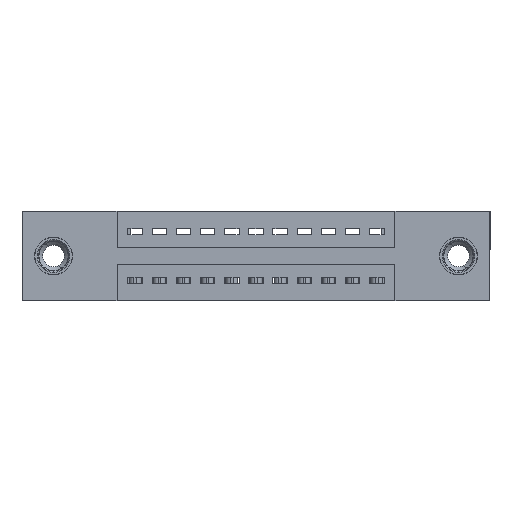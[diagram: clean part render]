
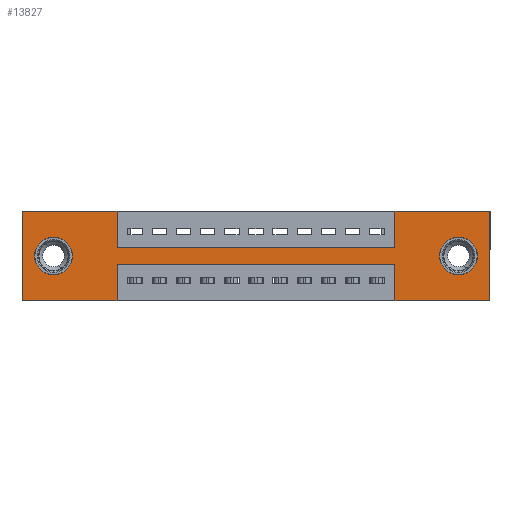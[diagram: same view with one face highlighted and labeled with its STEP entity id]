
A CAD part, front view. The second image highlights one B-rep face of the part: STEP entity #13827.
In plain terms, the highlighted planar face has unit normal (0, -1, 0).
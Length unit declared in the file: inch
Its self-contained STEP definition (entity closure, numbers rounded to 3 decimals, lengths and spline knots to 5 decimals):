
#145 = CARTESIAN_POINT ( 'NONE',  ( 0., 0., -0.37 ) ) ;
#347 = ORIENTED_EDGE ( 'NONE', *, *, #14612, .T. ) ;
#535 = CARTESIAN_POINT ( 'NONE',  ( 1.805, 0., -0.185 ) ) ;
#588 = LINE ( 'NONE', #3285, #9502 ) ;
#739 = ORIENTED_EDGE ( 'NONE', *, *, #3452, .F. ) ;
#837 = EDGE_CURVE ( 'NONE', #3271, #6116, #16174, .T. ) ;
#851 = FACE_BOUND ( 'NONE', #16151, .T. ) ;
#891 = VERTEX_POINT ( 'NONE', #9040 ) ;
#988 = AXIS2_PLACEMENT_3D ( 'NONE', #5003, #3527, #16851 ) ;
#1136 = EDGE_CURVE ( 'NONE', #15679, #12880, #14702, .T. ) ;
#1168 = ORIENTED_EDGE ( 'NONE', *, *, #8587, .F. ) ;
#1301 = ORIENTED_EDGE ( 'NONE', *, *, #837, .F. ) ;
#1637 = CIRCLE ( 'NONE', #9508, 0.078 ) ;
#1881 = DIRECTION ( 'NONE',  ( 0., 1., 0. ) ) ;
#2131 = LINE ( 'NONE', #10244, #5858 ) ;
#2221 = DIRECTION ( 'NONE',  ( 0., 0., 1. ) ) ;
#2283 = VERTEX_POINT ( 'NONE', #6442 ) ;
#2339 = DIRECTION ( 'NONE',  ( 1., 0., 0. ) ) ;
#2840 = CARTESIAN_POINT ( 'NONE',  ( 0.3925, 0., -0.22 ) ) ;
#2903 = VERTEX_POINT ( 'NONE', #14888 ) ;
#2966 = CIRCLE ( 'NONE', #988, 0.078 ) ;
#3119 = CARTESIAN_POINT ( 'NONE',  ( 1.5425, 0., 0. ) ) ;
#3271 = VERTEX_POINT ( 'NONE', #4551 ) ;
#3276 = VERTEX_POINT ( 'NONE', #3298 ) ;
#3285 = CARTESIAN_POINT ( 'NONE',  ( 0.3925, 0., -0.15 ) ) ;
#3298 = CARTESIAN_POINT ( 'NONE',  ( 1.935, 0., -0.37 ) ) ;
#3301 = VERTEX_POINT ( 'NONE', #7769 ) ;
#3452 = EDGE_CURVE ( 'NONE', #891, #11376, #14467, .T. ) ;
#3463 = VECTOR ( 'NONE', #6060, 39.37008 ) ;
#3464 = LINE ( 'NONE', #3119, #4306 ) ;
#3527 = DIRECTION ( 'NONE',  ( 0., 1., 0. ) ) ;
#3656 = CARTESIAN_POINT ( 'NONE',  ( 0., 0., 0. ) ) ;
#3719 = ORIENTED_EDGE ( 'NONE', *, *, #5097, .F. ) ;
#3980 = EDGE_CURVE ( 'NONE', #2903, #5369, #588, .T. ) ;
#4088 = AXIS2_PLACEMENT_3D ( 'NONE', #11231, #12557, #16885 ) ;
#4231 = VECTOR ( 'NONE', #11569, 39.37008 ) ;
#4254 = DIRECTION ( 'NONE',  ( 0., 0., 1. ) ) ;
#4306 = VECTOR ( 'NONE', #4254, 39.37008 ) ;
#4396 = CARTESIAN_POINT ( 'NONE',  ( 0.3925, 0., -0.22 ) ) ;
#4400 = ORIENTED_EDGE ( 'NONE', *, *, #10268, .F. ) ;
#4551 = CARTESIAN_POINT ( 'NONE',  ( 0., 0., 0. ) ) ;
#4624 = VECTOR ( 'NONE', #12164, 39.37008 ) ;
#4629 = ORIENTED_EDGE ( 'NONE', *, *, #10892, .F. ) ;
#4872 = PLANE ( 'NONE',  #4088 ) ;
#5003 = CARTESIAN_POINT ( 'NONE',  ( 0.13, 0., -0.185 ) ) ;
#5087 = VECTOR ( 'NONE', #11631, 39.37008 ) ;
#5097 = EDGE_CURVE ( 'NONE', #11376, #3301, #11520, .T. ) ;
#5207 = CARTESIAN_POINT ( 'NONE',  ( 0.13, 0., -0.107 ) ) ;
#5263 = EDGE_CURVE ( 'NONE', #5369, #9831, #3464, .T. ) ;
#5315 = ORIENTED_EDGE ( 'NONE', *, *, #3980, .F. ) ;
#5369 = VERTEX_POINT ( 'NONE', #14026 ) ;
#5533 = VERTEX_POINT ( 'NONE', #7698 ) ;
#5627 = DIRECTION ( 'NONE',  ( -1., 0., 0. ) ) ;
#5721 = CARTESIAN_POINT ( 'NONE',  ( 1.805, 0., -0.185 ) ) ;
#5858 = VECTOR ( 'NONE', #11624, 39.37008 ) ;
#5893 = ORIENTED_EDGE ( 'NONE', *, *, #1136, .T. ) ;
#5897 = CARTESIAN_POINT ( 'NONE',  ( 1.5425, 0., 0. ) ) ;
#5966 = DIRECTION ( 'NONE',  ( 0., 0., -1. ) ) ;
#6060 = DIRECTION ( 'NONE',  ( 0., 0., -1. ) ) ;
#6116 = VERTEX_POINT ( 'NONE', #10850 ) ;
#6301 = VERTEX_POINT ( 'NONE', #16018 ) ;
#6442 = CARTESIAN_POINT ( 'NONE',  ( 0., 0., -0.37 ) ) ;
#6686 = DIRECTION ( 'NONE',  ( 0., 0., -1. ) ) ;
#7029 = EDGE_CURVE ( 'NONE', #16158, #5533, #15606, .T. ) ;
#7040 = CARTESIAN_POINT ( 'NONE',  ( 1.935, 0., 0. ) ) ;
#7057 = CARTESIAN_POINT ( 'NONE',  ( 1.5425, 0., -0.37 ) ) ;
#7170 = VECTOR ( 'NONE', #2221, 39.37008 ) ;
#7318 = FACE_BOUND ( 'NONE', #10980, .T. ) ;
#7380 = CARTESIAN_POINT ( 'NONE',  ( 0., 0., 0. ) ) ;
#7698 = CARTESIAN_POINT ( 'NONE',  ( 1.805, 0., -0.263 ) ) ;
#7764 = EDGE_CURVE ( 'NONE', #6301, #891, #8377, .T. ) ;
#7769 = CARTESIAN_POINT ( 'NONE',  ( 0.3925, 0., -0.37 ) ) ;
#8266 = CARTESIAN_POINT ( 'NONE',  ( 0.13, 0., -0.185 ) ) ;
#8377 = LINE ( 'NONE', #7057, #13283 ) ;
#8478 = CARTESIAN_POINT ( 'NONE',  ( 0., 0., 0. ) ) ;
#8587 = EDGE_CURVE ( 'NONE', #3301, #2283, #17018, .T. ) ;
#8606 = LINE ( 'NONE', #7380, #7170 ) ;
#8655 = VECTOR ( 'NONE', #6686, 39.37008 ) ;
#9040 = CARTESIAN_POINT ( 'NONE',  ( 1.5425, 0., -0.22 ) ) ;
#9500 = CARTESIAN_POINT ( 'NONE',  ( 0.13, 0., -0.263 ) ) ;
#9502 = VECTOR ( 'NONE', #11256, 39.37008 ) ;
#9508 = AXIS2_PLACEMENT_3D ( 'NONE', #535, #1881, #5966 ) ;
#9686 = DIRECTION ( 'NONE',  ( 0., 0., 1. ) ) ;
#9746 = DIRECTION ( 'NONE',  ( 0., 0., -1. ) ) ;
#9831 = VERTEX_POINT ( 'NONE', #5897 ) ;
#10244 = CARTESIAN_POINT ( 'NONE',  ( 1.935, 0., 0. ) ) ;
#10268 = EDGE_CURVE ( 'NONE', #6116, #2903, #10880, .T. ) ;
#10292 = ORIENTED_EDGE ( 'NONE', *, *, #16569, .T. ) ;
#10850 = CARTESIAN_POINT ( 'NONE',  ( 0.3925, 0., 0. ) ) ;
#10880 = LINE ( 'NONE', #13743, #3463 ) ;
#10892 = EDGE_CURVE ( 'NONE', #2283, #3271, #8606, .T. ) ;
#10980 = EDGE_LOOP ( 'NONE', ( #5893, #10292 ) ) ;
#11017 = DIRECTION ( 'NONE',  ( 0., 0., 1. ) ) ;
#11073 = DIRECTION ( 'NONE',  ( 0., 1., 0. ) ) ;
#11231 = CARTESIAN_POINT ( 'NONE',  ( 0., 0., -0.37 ) ) ;
#11256 = DIRECTION ( 'NONE',  ( 1., 0., 0. ) ) ;
#11376 = VERTEX_POINT ( 'NONE', #4396 ) ;
#11520 = LINE ( 'NONE', #13198, #8655 ) ;
#11569 = DIRECTION ( 'NONE',  ( -1., 0., 0. ) ) ;
#11624 = DIRECTION ( 'NONE',  ( 0., 0., -1. ) ) ;
#11631 = DIRECTION ( 'NONE',  ( 1., 0., 0. ) ) ;
#11719 = VERTEX_POINT ( 'NONE', #7040 ) ;
#11751 = EDGE_CURVE ( 'NONE', #9831, #11719, #14333, .T. ) ;
#11904 = EDGE_LOOP ( 'NONE', ( #3719, #739, #15040, #16695, #15784, #16623, #16529, #5315, #4400, #1301, #4629, #1168 ) ) ;
#12164 = DIRECTION ( 'NONE',  ( -1., 0., 0. ) ) ;
#12221 = DIRECTION ( 'NONE',  ( 0., 1., 0. ) ) ;
#12518 = EDGE_CURVE ( 'NONE', #11719, #3276, #2131, .T. ) ;
#12557 = DIRECTION ( 'NONE',  ( 0., -1., 0. ) ) ;
#12834 = AXIS2_PLACEMENT_3D ( 'NONE', #8266, #12221, #9686 ) ;
#12880 = VERTEX_POINT ( 'NONE', #9500 ) ;
#12990 = CARTESIAN_POINT ( 'NONE',  ( 0., 0., -0.37 ) ) ;
#13198 = CARTESIAN_POINT ( 'NONE',  ( 0.3925, 0., -0.37 ) ) ;
#13283 = VECTOR ( 'NONE', #11017, 39.37008 ) ;
#13743 = CARTESIAN_POINT ( 'NONE',  ( 0.3925, 0., 0. ) ) ;
#13827 = ADVANCED_FACE ( 'NONE', ( #851, #7318, #13888 ), #4872, .T. ) ;
#13888 = FACE_OUTER_BOUND ( 'NONE', #11904, .T. ) ;
#14006 = AXIS2_PLACEMENT_3D ( 'NONE', #5721, #11073, #9746 ) ;
#14026 = CARTESIAN_POINT ( 'NONE',  ( 1.5425, 0., -0.15 ) ) ;
#14058 = EDGE_CURVE ( 'NONE', #3276, #6301, #16768, .T. ) ;
#14333 = LINE ( 'NONE', #8478, #5087 ) ;
#14467 = LINE ( 'NONE', #2840, #16131 ) ;
#14612 = EDGE_CURVE ( 'NONE', #5533, #16158, #1637, .T. ) ;
#14702 = CIRCLE ( 'NONE', #12834, 0.078 ) ;
#14888 = CARTESIAN_POINT ( 'NONE',  ( 0.3925, 0., -0.15 ) ) ;
#15040 = ORIENTED_EDGE ( 'NONE', *, *, #7764, .F. ) ;
#15606 = CIRCLE ( 'NONE', #14006, 0.078 ) ;
#15653 = CARTESIAN_POINT ( 'NONE',  ( 1.805, 0., -0.107 ) ) ;
#15679 = VERTEX_POINT ( 'NONE', #5207 ) ;
#15721 = ORIENTED_EDGE ( 'NONE', *, *, #7029, .T. ) ;
#15784 = ORIENTED_EDGE ( 'NONE', *, *, #12518, .F. ) ;
#16018 = CARTESIAN_POINT ( 'NONE',  ( 1.5425, 0., -0.37 ) ) ;
#16131 = VECTOR ( 'NONE', #5627, 39.37008 ) ;
#16151 = EDGE_LOOP ( 'NONE', ( #15721, #347 ) ) ;
#16158 = VERTEX_POINT ( 'NONE', #15653 ) ;
#16174 = LINE ( 'NONE', #3656, #16571 ) ;
#16529 = ORIENTED_EDGE ( 'NONE', *, *, #5263, .F. ) ;
#16569 = EDGE_CURVE ( 'NONE', #12880, #15679, #2966, .T. ) ;
#16571 = VECTOR ( 'NONE', #2339, 39.37008 ) ;
#16623 = ORIENTED_EDGE ( 'NONE', *, *, #11751, .F. ) ;
#16695 = ORIENTED_EDGE ( 'NONE', *, *, #14058, .F. ) ;
#16768 = LINE ( 'NONE', #145, #4624 ) ;
#16851 = DIRECTION ( 'NONE',  ( 0., 0., 1. ) ) ;
#16885 = DIRECTION ( 'NONE',  ( 0., 0., -1. ) ) ;
#17018 = LINE ( 'NONE', #12990, #4231 ) ;
